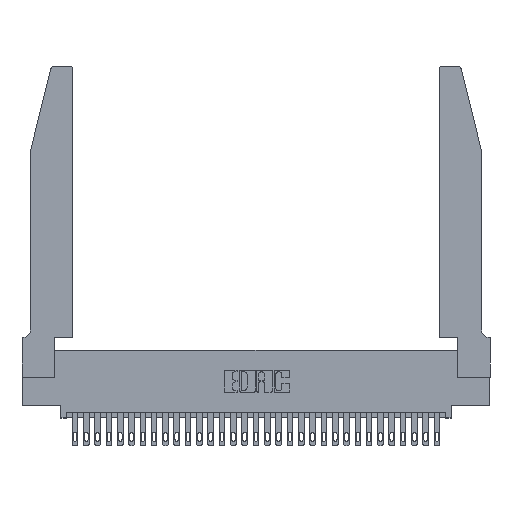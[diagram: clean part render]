
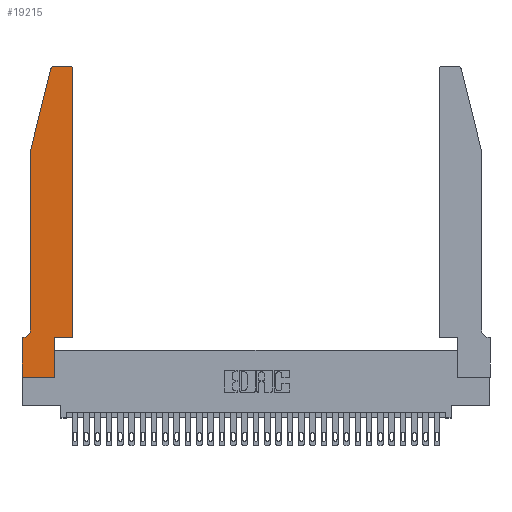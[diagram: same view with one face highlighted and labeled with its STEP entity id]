
A CAD part, top view. The second image highlights one B-rep face of the part: STEP entity #19215.
In plain terms, the highlighted planar face has unit normal (0, 0, 1).
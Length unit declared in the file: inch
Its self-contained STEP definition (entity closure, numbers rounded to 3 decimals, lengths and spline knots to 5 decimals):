
#391 = DIRECTION ( 'NONE',  ( -1., 0., 0. ) ) ;
#518 = CARTESIAN_POINT ( 'NONE',  ( 0., 0.35, 0.37 ) ) ;
#519 = ORIENTED_EDGE ( 'NONE', *, *, #17195, .T. ) ;
#1484 = DIRECTION ( 'NONE',  ( 0., -1., 0. ) ) ;
#1553 = ORIENTED_EDGE ( 'NONE', *, *, #17963, .T. ) ;
#1911 = CARTESIAN_POINT ( 'NONE',  ( 0.0055, 0.35, 0.37 ) ) ;
#1913 = VERTEX_POINT ( 'NONE', #4037 ) ;
#2135 = LINE ( 'NONE', #26229, #30662 ) ;
#2159 = EDGE_LOOP ( 'NONE', ( #21573, #519, #23117, #16890, #22563, #24330, #10357, #15279, #11415, #7046, #1553, #18634 ) ) ;
#2605 = LINE ( 'NONE', #6938, #16163 ) ;
#3029 = DIRECTION ( 'NONE',  ( 0., 0., 1. ) ) ;
#3579 = VERTEX_POINT ( 'NONE', #1911 ) ;
#3697 = LINE ( 'NONE', #5192, #16081 ) ;
#3843 = VERTEX_POINT ( 'NONE', #11175 ) ;
#4037 = CARTESIAN_POINT ( 'NONE',  ( 0.4505, 0.35, 0.37 ) ) ;
#5192 = CARTESIAN_POINT ( 'NONE',  ( 0.2865, 0.35, 0.37 ) ) ;
#5344 = VERTEX_POINT ( 'NONE', #5859 ) ;
#5859 = CARTESIAN_POINT ( 'NONE',  ( 0.25487, 2.72718, 0.37 ) ) ;
#6609 = DIRECTION ( 'NONE',  ( -1., 0., 0. ) ) ;
#6625 = DIRECTION ( 'NONE',  ( 1., 0., 0. ) ) ;
#6938 = CARTESIAN_POINT ( 'NONE',  ( 0., 0., 0.37 ) ) ;
#7046 = ORIENTED_EDGE ( 'NONE', *, *, #11326, .T. ) ;
#7564 = DIRECTION ( 'NONE',  ( 0., -1., 0. ) ) ;
#8204 = EDGE_CURVE ( 'NONE', #5344, #8799, #29380, .T. ) ;
#8357 = CARTESIAN_POINT ( 'NONE',  ( 0.4205, 2.72, 0.37 ) ) ;
#8598 = VECTOR ( 'NONE', #8916, 39.37008 ) ;
#8799 = VERTEX_POINT ( 'NONE', #14095 ) ;
#8916 = DIRECTION ( 'NONE',  ( -0.239, -0.971, 0. ) ) ;
#8988 = DIRECTION ( 'NONE',  ( 1., 0., 0. ) ) ;
#9422 = DIRECTION ( 'NONE',  ( 1., 0., 0. ) ) ;
#9663 = EDGE_CURVE ( 'NONE', #8799, #24631, #23482, .T. ) ;
#10041 = EDGE_CURVE ( 'NONE', #24631, #3579, #22303, .T. ) ;
#10279 = CARTESIAN_POINT ( 'NONE',  ( 0., 0., 0.37 ) ) ;
#10357 = ORIENTED_EDGE ( 'NONE', *, *, #14052, .T. ) ;
#10638 = AXIS2_PLACEMENT_3D ( 'NONE', #8357, #23332, #8988 ) ;
#11080 = FACE_OUTER_BOUND ( 'NONE', #2159, .T. ) ;
#11175 = CARTESIAN_POINT ( 'NONE',  ( 0.4205, 2.75, 0.37 ) ) ;
#11293 = VECTOR ( 'NONE', #6609, 39.37008 ) ;
#11326 = EDGE_CURVE ( 'NONE', #31766, #1913, #2135, .T. ) ;
#11413 = VECTOR ( 'NONE', #23334, 39.37008 ) ;
#11415 = ORIENTED_EDGE ( 'NONE', *, *, #25769, .T. ) ;
#12082 = LINE ( 'NONE', #16337, #11293 ) ;
#12537 = VERTEX_POINT ( 'NONE', #15542 ) ;
#12762 = DIRECTION ( 'NONE',  ( 0., 0., -1. ) ) ;
#13791 = EDGE_CURVE ( 'NONE', #16921, #3843, #30848, .T. ) ;
#13820 = CARTESIAN_POINT ( 'NONE',  ( 0., 0.35, 0.37 ) ) ;
#13919 = CARTESIAN_POINT ( 'NONE',  ( 0.0755, 0.42, 0.37 ) ) ;
#13964 = DIRECTION ( 'NONE',  ( 0., 0., 1. ) ) ;
#14052 = EDGE_CURVE ( 'NONE', #22467, #23267, #23549, .T. ) ;
#14095 = CARTESIAN_POINT ( 'NONE',  ( 0.0755, 2., 0.37 ) ) ;
#15279 = ORIENTED_EDGE ( 'NONE', *, *, #19015, .T. ) ;
#15542 = CARTESIAN_POINT ( 'NONE',  ( 0.2865, 0., 0.37 ) ) ;
#15662 = LINE ( 'NONE', #18186, #11413 ) ;
#16081 = VECTOR ( 'NONE', #24639, 39.37008 ) ;
#16083 = CARTESIAN_POINT ( 'NONE',  ( 0.4505, 0.35, 0.37 ) ) ;
#16163 = VECTOR ( 'NONE', #9422, 39.37008 ) ;
#16337 = CARTESIAN_POINT ( 'NONE',  ( 0.0755, 0.35, 0.37 ) ) ;
#16705 = AXIS2_PLACEMENT_3D ( 'NONE', #25907, #13964, #6625 ) ;
#16890 = ORIENTED_EDGE ( 'NONE', *, *, #9663, .T. ) ;
#16921 = VERTEX_POINT ( 'NONE', #29661 ) ;
#16972 = VECTOR ( 'NONE', #1484, 39.37008 ) ;
#17195 = EDGE_CURVE ( 'NONE', #21235, #5344, #23150, .T. ) ;
#17343 = LINE ( 'NONE', #16083, #29255 ) ;
#17709 = CARTESIAN_POINT ( 'NONE',  ( 0.0055, 0.42, 0.37 ) ) ;
#17963 = EDGE_CURVE ( 'NONE', #1913, #16921, #17343, .T. ) ;
#17998 = CARTESIAN_POINT ( 'NONE',  ( 0.0755, 2., 0.37 ) ) ;
#18186 = CARTESIAN_POINT ( 'NONE',  ( 0.2605, 2.75, 0.37 ) ) ;
#18245 = PLANE ( 'NONE',  #29059 ) ;
#18634 = ORIENTED_EDGE ( 'NONE', *, *, #13791, .T. ) ;
#18674 = CARTESIAN_POINT ( 'NONE',  ( 0.0755, 2., 0.37 ) ) ;
#19015 = EDGE_CURVE ( 'NONE', #23267, #12537, #2605, .T. ) ;
#19043 = DIRECTION ( 'NONE',  ( 1., 0., 0. ) ) ;
#19215 = ADVANCED_FACE ( 'NONE', ( #11080 ), #18245, .T. ) ;
#21111 = EDGE_CURVE ( 'NONE', #3843, #21235, #15662, .T. ) ;
#21235 = VERTEX_POINT ( 'NONE', #25370 ) ;
#21573 = ORIENTED_EDGE ( 'NONE', *, *, #21111, .T. ) ;
#22180 = CARTESIAN_POINT ( 'NONE',  ( 0., 0., 0.37 ) ) ;
#22303 = CIRCLE ( 'NONE', #26637, 0.07 ) ;
#22467 = VERTEX_POINT ( 'NONE', #13820 ) ;
#22563 = ORIENTED_EDGE ( 'NONE', *, *, #10041, .T. ) ;
#23038 = DIRECTION ( 'NONE',  ( 0., 1., 0. ) ) ;
#23066 = DIRECTION ( 'NONE',  ( 1., 0., 0. ) ) ;
#23117 = ORIENTED_EDGE ( 'NONE', *, *, #8204, .T. ) ;
#23150 = CIRCLE ( 'NONE', #16705, 0.03 ) ;
#23237 = CARTESIAN_POINT ( 'NONE',  ( 0.2865, 0.35, 0.37 ) ) ;
#23267 = VERTEX_POINT ( 'NONE', #10279 ) ;
#23332 = DIRECTION ( 'NONE',  ( 0., 0., 1. ) ) ;
#23334 = DIRECTION ( 'NONE',  ( -1., 0., 0. ) ) ;
#23482 = LINE ( 'NONE', #18674, #16972 ) ;
#23549 = LINE ( 'NONE', #22180, #26254 ) ;
#24330 = ORIENTED_EDGE ( 'NONE', *, *, #27507, .T. ) ;
#24631 = VERTEX_POINT ( 'NONE', #13919 ) ;
#24639 = DIRECTION ( 'NONE',  ( 0., 1., 0. ) ) ;
#25370 = CARTESIAN_POINT ( 'NONE',  ( 0.284, 2.75, 0.37 ) ) ;
#25769 = EDGE_CURVE ( 'NONE', #12537, #31766, #3697, .T. ) ;
#25907 = CARTESIAN_POINT ( 'NONE',  ( 0.284, 2.72, 0.37 ) ) ;
#26229 = CARTESIAN_POINT ( 'NONE',  ( 0.4505, 0.35, 0.37 ) ) ;
#26254 = VECTOR ( 'NONE', #7564, 39.37008 ) ;
#26637 = AXIS2_PLACEMENT_3D ( 'NONE', #17709, #12762, #391 ) ;
#27507 = EDGE_CURVE ( 'NONE', #3579, #22467, #12082, .T. ) ;
#29059 = AXIS2_PLACEMENT_3D ( 'NONE', #518, #3029, #23066 ) ;
#29255 = VECTOR ( 'NONE', #23038, 39.37008 ) ;
#29380 = LINE ( 'NONE', #17998, #8598 ) ;
#29661 = CARTESIAN_POINT ( 'NONE',  ( 0.4505, 2.72, 0.37 ) ) ;
#30662 = VECTOR ( 'NONE', #19043, 39.37008 ) ;
#30848 = CIRCLE ( 'NONE', #10638, 0.03 ) ;
#31766 = VERTEX_POINT ( 'NONE', #23237 ) ;
